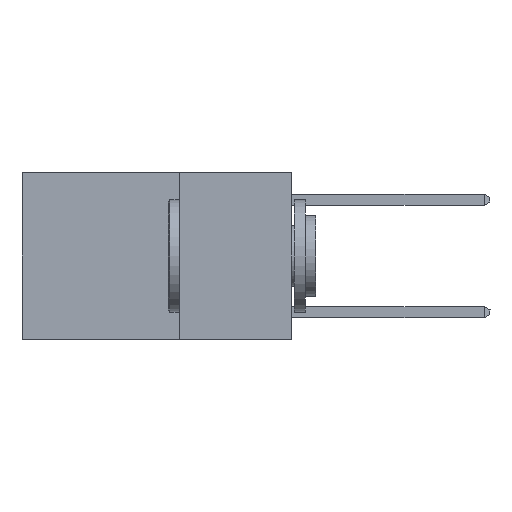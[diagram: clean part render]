
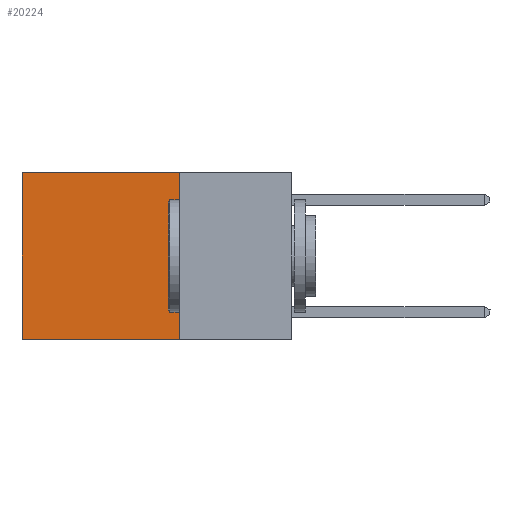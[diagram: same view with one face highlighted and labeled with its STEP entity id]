
A CAD part, left-side view. The second image highlights one B-rep face of the part: STEP entity #20224.
In plain terms, the highlighted planar face has unit normal (-1, 0, 0).
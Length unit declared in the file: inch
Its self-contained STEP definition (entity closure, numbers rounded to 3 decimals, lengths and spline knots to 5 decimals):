
#895 = AXIS2_PLACEMENT_3D ( 'NONE', #10158, #15236, #4995 ) ;
#1559 = DIRECTION ( 'NONE',  ( 0., 1., 0. ) ) ;
#1650 = EDGE_LOOP ( 'NONE', ( #15030, #10779, #3975, #1794 ) ) ;
#1794 = ORIENTED_EDGE ( 'NONE', *, *, #16330, .T. ) ;
#1815 = VERTEX_POINT ( 'NONE', #20824 ) ;
#1915 = EDGE_CURVE ( 'NONE', #1815, #12928, #15674, .T. ) ;
#1983 = VECTOR ( 'NONE', #2498, 39.37008 ) ;
#2498 = DIRECTION ( 'NONE',  ( 0., 1., 0. ) ) ;
#2835 = DIRECTION ( 'NONE',  ( 0., 0., -1. ) ) ;
#3384 = CARTESIAN_POINT ( 'NONE',  ( 0.2625, 0.25, 0. ) ) ;
#3394 = EDGE_CURVE ( 'NONE', #5419, #12928, #11147, .T. ) ;
#3697 = EDGE_CURVE ( 'NONE', #10903, #1815, #13218, .T. ) ;
#3975 = ORIENTED_EDGE ( 'NONE', *, *, #3697, .F. ) ;
#4915 = PLANE ( 'NONE',  #895 ) ;
#4995 = DIRECTION ( 'NONE',  ( 0., 0., -1. ) ) ;
#5419 = VERTEX_POINT ( 'NONE', #19081 ) ;
#7506 = LINE ( 'NONE', #3384, #11549 ) ;
#9243 = VECTOR ( 'NONE', #21454, 39.37008 ) ;
#9865 = CARTESIAN_POINT ( 'NONE',  ( 0.2625, 0.25, 0. ) ) ;
#10158 = CARTESIAN_POINT ( 'NONE',  ( 0.2625, 0.25, 0. ) ) ;
#10779 = ORIENTED_EDGE ( 'NONE', *, *, #1915, .F. ) ;
#10903 = VERTEX_POINT ( 'NONE', #21010 ) ;
#11141 = CARTESIAN_POINT ( 'NONE',  ( 0.2625, 0.25, -0.37 ) ) ;
#11147 = LINE ( 'NONE', #14845, #18953 ) ;
#11549 = VECTOR ( 'NONE', #1559, 39.37008 ) ;
#12928 = VERTEX_POINT ( 'NONE', #12968 ) ;
#12968 = CARTESIAN_POINT ( 'NONE',  ( 0.2625, 0.6, -0.37 ) ) ;
#13218 = LINE ( 'NONE', #9865, #9243 ) ;
#14845 = CARTESIAN_POINT ( 'NONE',  ( 0.2625, 0.6, 0. ) ) ;
#15030 = ORIENTED_EDGE ( 'NONE', *, *, #3394, .T. ) ;
#15236 = DIRECTION ( 'NONE',  ( 1., 0., 0. ) ) ;
#15674 = LINE ( 'NONE', #11141, #1983 ) ;
#16330 = EDGE_CURVE ( 'NONE', #10903, #5419, #7506, .T. ) ;
#18953 = VECTOR ( 'NONE', #2835, 39.37008 ) ;
#19081 = CARTESIAN_POINT ( 'NONE',  ( 0.2625, 0.6, 0. ) ) ;
#20224 = ADVANCED_FACE ( 'NONE', ( #20696 ), #4915, .F. ) ;
#20696 = FACE_OUTER_BOUND ( 'NONE', #1650, .T. ) ;
#20824 = CARTESIAN_POINT ( 'NONE',  ( 0.2625, 0.25, -0.37 ) ) ;
#21010 = CARTESIAN_POINT ( 'NONE',  ( 0.2625, 0.25, 0. ) ) ;
#21454 = DIRECTION ( 'NONE',  ( 0., 0., -1. ) ) ;
